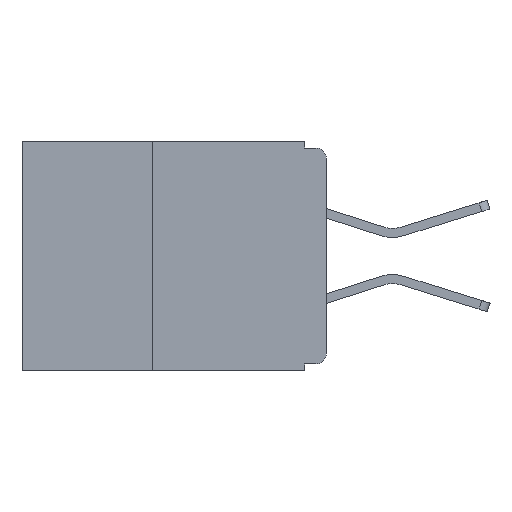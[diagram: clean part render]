
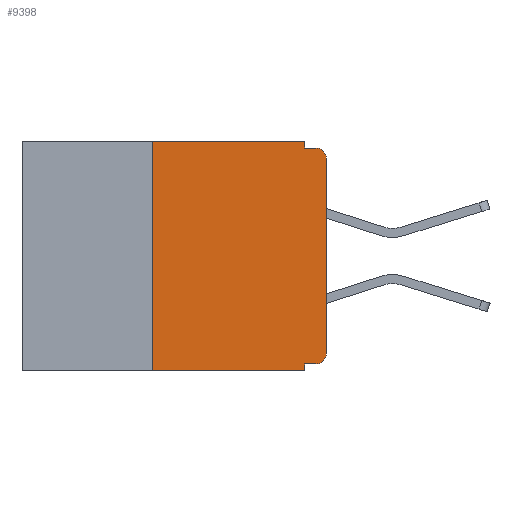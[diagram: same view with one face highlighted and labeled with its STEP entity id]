
A CAD part, left-side view. The second image highlights one B-rep face of the part: STEP entity #9398.
In plain terms, the highlighted planar face has unit normal (-1, 0, 0).
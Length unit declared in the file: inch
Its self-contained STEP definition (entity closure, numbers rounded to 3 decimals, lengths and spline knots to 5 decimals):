
#416 = ORIENTED_EDGE ( 'NONE', *, *, #8478, .T. ) ;
#485 = LINE ( 'NONE', #4346, #2880 ) ;
#629 = ORIENTED_EDGE ( 'NONE', *, *, #3268, .T. ) ;
#745 = VECTOR ( 'NONE', #6046, 39.37008 ) ;
#762 = CARTESIAN_POINT ( 'NONE',  ( 0., 0.437, -0.33 ) ) ;
#825 = VERTEX_POINT ( 'NONE', #3537 ) ;
#1013 = VERTEX_POINT ( 'NONE', #9799 ) ;
#1016 = LINE ( 'NONE', #6000, #7606 ) ;
#1142 = EDGE_CURVE ( 'NONE', #6593, #1013, #5299, .T. ) ;
#1255 = EDGE_CURVE ( 'NONE', #4602, #825, #485, .T. ) ;
#1403 = CIRCLE ( 'NONE', #9917, 0.015 ) ;
#1412 = LINE ( 'NONE', #11027, #6507 ) ;
#1598 = DIRECTION ( 'NONE',  ( 0., -1., 0. ) ) ;
#1679 = VECTOR ( 'NONE', #2150, 39.37008 ) ;
#1731 = ORIENTED_EDGE ( 'NONE', *, *, #7781, .F. ) ;
#1754 = DIRECTION ( 'NONE',  ( 0., 1., 0. ) ) ;
#1955 = DIRECTION ( 'NONE',  ( 0., 0., 1. ) ) ;
#1997 = ORIENTED_EDGE ( 'NONE', *, *, #7906, .T. ) ;
#2042 = ORIENTED_EDGE ( 'NONE', *, *, #4751, .F. ) ;
#2150 = DIRECTION ( 'NONE',  ( 0., -1., 0. ) ) ;
#2442 = CARTESIAN_POINT ( 'NONE',  ( 0., 0.437, 0. ) ) ;
#2710 = FACE_OUTER_BOUND ( 'NONE', #7886, .T. ) ;
#2790 = DIRECTION ( 'NONE',  ( 0., 0., -1. ) ) ;
#2851 = DIRECTION ( 'NONE',  ( 0., 0., -1. ) ) ;
#2880 = VECTOR ( 'NONE', #1754, 39.37008 ) ;
#2907 = CARTESIAN_POINT ( 'NONE',  ( 0., 0., -0.025 ) ) ;
#3245 = DIRECTION ( 'NONE',  ( 1., 0., 0. ) ) ;
#3268 = EDGE_CURVE ( 'NONE', #6549, #1013, #10156, .T. ) ;
#3339 = ORIENTED_EDGE ( 'NONE', *, *, #7555, .F. ) ;
#3504 = CARTESIAN_POINT ( 'NONE',  ( 0., 0.015, -0.32 ) ) ;
#3537 = CARTESIAN_POINT ( 'NONE',  ( 0., 0.031, -0.32 ) ) ;
#3616 = CARTESIAN_POINT ( 'NONE',  ( 0., 0., 0. ) ) ;
#3762 = CARTESIAN_POINT ( 'NONE',  ( 0., 0., -0.305 ) ) ;
#3841 = VERTEX_POINT ( 'NONE', #10861 ) ;
#3938 = CARTESIAN_POINT ( 'NONE',  ( 0., 0.25, -0.33 ) ) ;
#4088 = VERTEX_POINT ( 'NONE', #9918 ) ;
#4104 = VERTEX_POINT ( 'NONE', #5638 ) ;
#4288 = DIRECTION ( 'NONE',  ( 0., 0., 1. ) ) ;
#4346 = CARTESIAN_POINT ( 'NONE',  ( 0., 0., -0.32 ) ) ;
#4519 = EDGE_CURVE ( 'NONE', #8283, #4088, #8136, .T. ) ;
#4602 = VERTEX_POINT ( 'NONE', #3504 ) ;
#4608 = CARTESIAN_POINT ( 'NONE',  ( 0., 0.031, -0.01 ) ) ;
#4751 = EDGE_CURVE ( 'NONE', #825, #4088, #7465, .T. ) ;
#4785 = AXIS2_PLACEMENT_3D ( 'NONE', #5588, #8970, #2851 ) ;
#5015 = DIRECTION ( 'NONE',  ( 0., 0., -1. ) ) ;
#5299 = LINE ( 'NONE', #9362, #7470 ) ;
#5588 = CARTESIAN_POINT ( 'NONE',  ( 0., 0.015, -0.025 ) ) ;
#5638 = CARTESIAN_POINT ( 'NONE',  ( 0., 0.25, 0. ) ) ;
#5662 = ORIENTED_EDGE ( 'NONE', *, *, #1142, .F. ) ;
#5979 = VECTOR ( 'NONE', #1598, 39.37008 ) ;
#6000 = CARTESIAN_POINT ( 'NONE',  ( 0., 0.25, -0.33 ) ) ;
#6036 = ORIENTED_EDGE ( 'NONE', *, *, #4519, .T. ) ;
#6046 = DIRECTION ( 'NONE',  ( 0., 0., -1. ) ) ;
#6507 = VECTOR ( 'NONE', #2790, 39.37008 ) ;
#6549 = VERTEX_POINT ( 'NONE', #2907 ) ;
#6593 = VERTEX_POINT ( 'NONE', #4608 ) ;
#6917 = EDGE_CURVE ( 'NONE', #8283, #4104, #1016, .T. ) ;
#6973 = VERTEX_POINT ( 'NONE', #3762 ) ;
#7363 = CARTESIAN_POINT ( 'NONE',  ( 0., 0.437, 0. ) ) ;
#7465 = LINE ( 'NONE', #7780, #745 ) ;
#7470 = VECTOR ( 'NONE', #9949, 39.37008 ) ;
#7514 = DIRECTION ( 'NONE',  ( -1., 0., 0. ) ) ;
#7555 = EDGE_CURVE ( 'NONE', #3841, #6593, #1412, .T. ) ;
#7606 = VECTOR ( 'NONE', #4288, 39.37008 ) ;
#7780 = CARTESIAN_POINT ( 'NONE',  ( 0., 0.031, -0.33 ) ) ;
#7781 = EDGE_CURVE ( 'NONE', #4104, #3841, #8662, .T. ) ;
#7886 = EDGE_LOOP ( 'NONE', ( #416, #629, #5662, #3339, #1731, #10841, #6036, #2042, #8006, #1997 ) ) ;
#7906 = EDGE_CURVE ( 'NONE', #4602, #6973, #1403, .T. ) ;
#8006 = ORIENTED_EDGE ( 'NONE', *, *, #1255, .F. ) ;
#8136 = LINE ( 'NONE', #762, #5979 ) ;
#8283 = VERTEX_POINT ( 'NONE', #3938 ) ;
#8467 = DIRECTION ( 'NONE',  ( 0., 0., -1. ) ) ;
#8478 = EDGE_CURVE ( 'NONE', #6973, #6549, #9454, .T. ) ;
#8649 = VECTOR ( 'NONE', #1955, 39.37008 ) ;
#8662 = LINE ( 'NONE', #7363, #1679 ) ;
#8970 = DIRECTION ( 'NONE',  ( -1., 0., 0. ) ) ;
#9292 = PLANE ( 'NONE',  #9618 ) ;
#9362 = CARTESIAN_POINT ( 'NONE',  ( 0., 0., -0.01 ) ) ;
#9398 = ADVANCED_FACE ( 'NONE', ( #2710 ), #9292, .F. ) ;
#9454 = LINE ( 'NONE', #3616, #8649 ) ;
#9618 = AXIS2_PLACEMENT_3D ( 'NONE', #2442, #3245, #5015 ) ;
#9799 = CARTESIAN_POINT ( 'NONE',  ( 0., 0.015, -0.01 ) ) ;
#9917 = AXIS2_PLACEMENT_3D ( 'NONE', #10975, #7514, #8467 ) ;
#9918 = CARTESIAN_POINT ( 'NONE',  ( 0., 0.031, -0.33 ) ) ;
#9949 = DIRECTION ( 'NONE',  ( 0., -1., 0. ) ) ;
#10156 = CIRCLE ( 'NONE', #4785, 0.015 ) ;
#10841 = ORIENTED_EDGE ( 'NONE', *, *, #6917, .F. ) ;
#10861 = CARTESIAN_POINT ( 'NONE',  ( 0., 0.031, 0. ) ) ;
#10975 = CARTESIAN_POINT ( 'NONE',  ( 0., 0.015, -0.305 ) ) ;
#11027 = CARTESIAN_POINT ( 'NONE',  ( 0., 0.031, 0. ) ) ;
